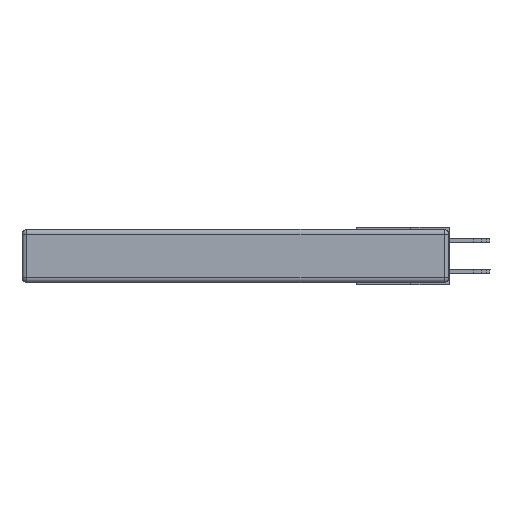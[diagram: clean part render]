
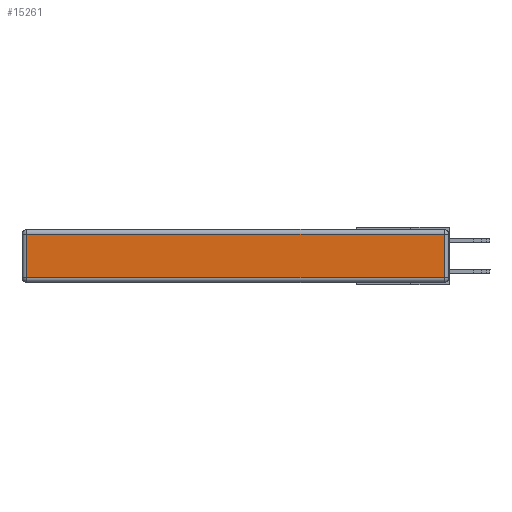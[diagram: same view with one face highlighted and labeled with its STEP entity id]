
A CAD part, left-side view. The second image highlights one B-rep face of the part: STEP entity #15261.
In plain terms, the highlighted planar face has unit normal (-1, 0, 0).
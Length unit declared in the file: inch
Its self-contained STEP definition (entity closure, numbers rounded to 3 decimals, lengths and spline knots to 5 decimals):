
#880 = LINE ( 'NONE', #15041, #2202 ) ;
#1430 = CARTESIAN_POINT ( 'NONE',  ( 0., 0., -0.313 ) ) ;
#1548 = CARTESIAN_POINT ( 'NONE',  ( 0., 0., -0.343 ) ) ;
#2202 = VECTOR ( 'NONE', #3489, 39.37008 ) ;
#2918 = FACE_OUTER_BOUND ( 'NONE', #16449, .T. ) ;
#3272 = CARTESIAN_POINT ( 'NONE',  ( 0., 2.72, -0.313 ) ) ;
#3489 = DIRECTION ( 'NONE',  ( 0., 0., -1. ) ) ;
#3875 = VECTOR ( 'NONE', #10994, 39.37008 ) ;
#4661 = ORIENTED_EDGE ( 'NONE', *, *, #10931, .T. ) ;
#5493 = CARTESIAN_POINT ( 'NONE',  ( 0., 0.03, -0.343 ) ) ;
#5838 = VERTEX_POINT ( 'NONE', #3272 ) ;
#6624 = DIRECTION ( 'NONE',  ( 0., 0., 1. ) ) ;
#7557 = CARTESIAN_POINT ( 'NONE',  ( 0., 2.75, -0.03 ) ) ;
#7601 = CARTESIAN_POINT ( 'NONE',  ( 0., 2.72, -0.03 ) ) ;
#8123 = DIRECTION ( 'NONE',  ( 0., -1., 0. ) ) ;
#8786 = CARTESIAN_POINT ( 'NONE',  ( 0., 0.03, -0.313 ) ) ;
#9900 = DIRECTION ( 'NONE',  ( -1., 0., 0. ) ) ;
#10845 = ORIENTED_EDGE ( 'NONE', *, *, #21708, .T. ) ;
#10931 = EDGE_CURVE ( 'NONE', #5838, #19437, #20637, .T. ) ;
#10994 = DIRECTION ( 'NONE',  ( 0., 1., 0. ) ) ;
#11072 = ORIENTED_EDGE ( 'NONE', *, *, #17895, .T. ) ;
#11795 = PLANE ( 'NONE',  #15388 ) ;
#12066 = LINE ( 'NONE', #5493, #15951 ) ;
#12509 = VECTOR ( 'NONE', #8123, 39.37008 ) ;
#13787 = DIRECTION ( 'NONE',  ( 0., 0., 1. ) ) ;
#14679 = CARTESIAN_POINT ( 'NONE',  ( 0., 0.03, -0.03 ) ) ;
#15041 = CARTESIAN_POINT ( 'NONE',  ( 0., 2.72, -0.343 ) ) ;
#15261 = ADVANCED_FACE ( 'NONE', ( #2918 ), #11795, .T. ) ;
#15388 = AXIS2_PLACEMENT_3D ( 'NONE', #1548, #9900, #6624 ) ;
#15951 = VECTOR ( 'NONE', #13787, 39.37008 ) ;
#15989 = EDGE_CURVE ( 'NONE', #19437, #21044, #12066, .T. ) ;
#16449 = EDGE_LOOP ( 'NONE', ( #4661, #20449, #10845, #11072 ) ) ;
#17895 = EDGE_CURVE ( 'NONE', #19486, #5838, #880, .T. ) ;
#19437 = VERTEX_POINT ( 'NONE', #8786 ) ;
#19486 = VERTEX_POINT ( 'NONE', #7601 ) ;
#20449 = ORIENTED_EDGE ( 'NONE', *, *, #15989, .T. ) ;
#20637 = LINE ( 'NONE', #1430, #12509 ) ;
#21044 = VERTEX_POINT ( 'NONE', #14679 ) ;
#21175 = LINE ( 'NONE', #7557, #3875 ) ;
#21708 = EDGE_CURVE ( 'NONE', #21044, #19486, #21175, .T. ) ;
